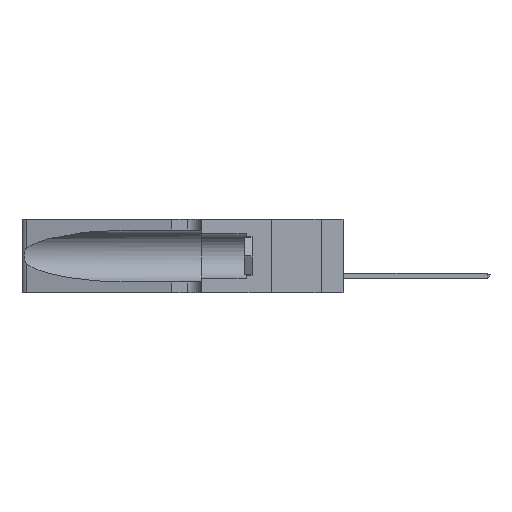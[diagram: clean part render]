
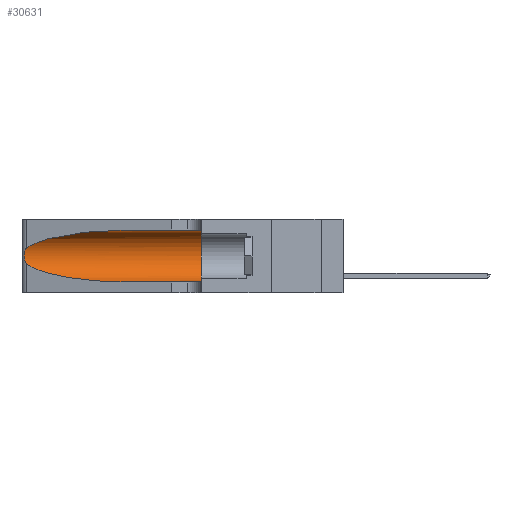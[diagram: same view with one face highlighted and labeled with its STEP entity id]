
A CAD part, left-side view. The second image highlights one B-rep face of the part: STEP entity #30631.
In plain terms, the highlighted cylindrical face has radius 3.308 mm (diameter 6.617 mm), a partial arc.
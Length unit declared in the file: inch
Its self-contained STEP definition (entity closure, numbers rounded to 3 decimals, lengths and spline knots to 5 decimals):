
#455 = ORIENTED_EDGE ( 'NONE', *, *, #36357, .T. ) ;
#565 = DIRECTION ( 'NONE',  ( 0., -1., 0. ) ) ;
#1757 = DIRECTION ( 'NONE',  ( 0., -1., 0. ) ) ;
#2036 = ORIENTED_EDGE ( 'NONE', *, *, #29687, .T. ) ;
#2436 = CARTESIAN_POINT ( 'NONE',  ( 0.26075, 1.23896, 0.178 ) ) ;
#4170 = CARTESIAN_POINT ( 'NONE',  ( 0.1305, 0.72297, 0.05475 ) ) ;
#4677 = CARTESIAN_POINT ( 'NONE',  ( 0.25555, 1.22993, 0.14849 ) ) ;
#5980 = CARTESIAN_POINT ( 'NONE',  ( 0.25789, 1.23486, 0.15765 ) ) ;
#6117 =( BOUNDED_CURVE ( )  B_SPLINE_CURVE ( 3, ( #19592, #31781, #31929, #4170 ),
 .UNSPECIFIED., .F., .T. ) 
 B_SPLINE_CURVE_WITH_KNOTS ( ( 4, 4 ),
 ( 3.44316, 4.71239 ),
 .UNSPECIFIED. ) 
 CURVE ( )  GEOMETRIC_REPRESENTATION_ITEM ( )  RATIONAL_B_SPLINE_CURVE ( ( 1., 0.87, 0.87, 1. ) ) 
 REPRESENTATION_ITEM ( '' )  );
#6506 = ORIENTED_EDGE ( 'NONE', *, *, #39464, .T. ) ;
#6916 = CARTESIAN_POINT ( 'NONE',  ( 0.25487, 1.22718, 0.22369 ) ) ;
#8922 = VERTEX_POINT ( 'NONE', #11744 ) ;
#9580 = CARTESIAN_POINT ( 'NONE',  ( 0.25639, 1.23184, 0.21858 ) ) ;
#11037 = CARTESIAN_POINT ( 'NONE',  ( 0.25856, 1.23593, 0.16098 ) ) ;
#11744 = CARTESIAN_POINT ( 'NONE',  ( 0.1305, 0.72297, 0.31525 ) ) ;
#13966 = CARTESIAN_POINT ( 'NONE',  ( 0.25487, 1.22718, 0.22369 ) ) ;
#14517 = CARTESIAN_POINT ( 'NONE',  ( 0.25854, 1.2359, 0.20912 ) ) ;
#14740 = VERTEX_POINT ( 'NONE', #47399 ) ;
#14896 = CARTESIAN_POINT ( 'NONE',  ( 0.26075, 1.23896, 0.19203 ) ) ;
#14962 = CARTESIAN_POINT ( 'NONE',  ( 0.2373, 1.15595, 0.28018 ) ) ;
#15559 = LINE ( 'NONE', #47718, #44718 ) ;
#15776 = VERTEX_POINT ( 'NONE', #25778 ) ;
#17312 = CARTESIAN_POINT ( 'NONE',  ( 0.1305, 0.72297, 0.05475 ) ) ;
#17535 = DIRECTION ( 'NONE',  ( 0., 0., 1. ) ) ;
#18070 = DIRECTION ( 'NONE',  ( 0., 0., -1. ) ) ;
#18720 = CARTESIAN_POINT ( 'NONE',  ( 0.26018, 1.23835, 0.19895 ) ) ;
#19592 = CARTESIAN_POINT ( 'NONE',  ( 0.25487, 1.22718, 0.14631 ) ) ;
#19971 = VERTEX_POINT ( 'NONE', #48031 ) ;
#20561 = CYLINDRICAL_SURFACE ( 'NONE', #24637, 0.13025 ) ;
#23439 = VECTOR ( 'NONE', #28861, 39.37008 ) ;
#24637 = AXIS2_PLACEMENT_3D ( 'NONE', #29691, #1757, #18070 ) ;
#24846 = FACE_OUTER_BOUND ( 'NONE', #45641, .T. ) ;
#25117 = CARTESIAN_POINT ( 'NONE',  ( 0.25487, 1.22718, 0.14631 ) ) ;
#25778 = CARTESIAN_POINT ( 'NONE',  ( 0.1305, 0.35, 0.31525 ) ) ;
#25941 = CIRCLE ( 'NONE', #40850, 0.13025 ) ;
#26321 = VERTEX_POINT ( 'NONE', #17312 ) ;
#26498 = CARTESIAN_POINT ( 'NONE',  ( 0.26017, 1.23833, 0.17102 ) ) ;
#27643 = ORIENTED_EDGE ( 'NONE', *, *, #34213, .F. ) ;
#28861 = DIRECTION ( 'NONE',  ( 0., -1., 0. ) ) ;
#29687 = EDGE_CURVE ( 'NONE', #8922, #14740, #35567, .T. ) ;
#29691 = CARTESIAN_POINT ( 'NONE',  ( 0.1305, 1.61858, 0.185 ) ) ;
#30631 = ADVANCED_FACE ( 'NONE', ( #24846 ), #20561, .F. ) ;
#30791 = CARTESIAN_POINT ( 'NONE',  ( 0.1305, 0.72297, 0.31525 ) ) ;
#31781 = CARTESIAN_POINT ( 'NONE',  ( 0.2373, 1.15595, 0.08982 ) ) ;
#31929 = CARTESIAN_POINT ( 'NONE',  ( 0.18966, 0.96281, 0.05475 ) ) ;
#34213 = EDGE_CURVE ( 'NONE', #8922, #15776, #15559, .T. ) ;
#34558 = ORIENTED_EDGE ( 'NONE', *, *, #35360, .F. ) ;
#35152 = CARTESIAN_POINT ( 'NONE',  ( 0.18966, 0.96281, 0.31525 ) ) ;
#35360 = EDGE_CURVE ( 'NONE', #15776, #44649, #25941, .T. ) ;
#35567 =( BOUNDED_CURVE ( )  B_SPLINE_CURVE ( 3, ( #30791, #35152, #14962, #6916 ),
 .UNSPECIFIED., .F., .T. ) 
 B_SPLINE_CURVE_WITH_KNOTS ( ( 4, 4 ),
 ( 1.5708, 2.84003 ),
 .UNSPECIFIED. ) 
 CURVE ( )  GEOMETRIC_REPRESENTATION_ITEM ( )  RATIONAL_B_SPLINE_CURVE ( ( 1., 0.87, 0.87, 1. ) ) 
 REPRESENTATION_ITEM ( '' )  );
#36357 = EDGE_CURVE ( 'NONE', #14740, #19971, #39429, .T. ) ;
#36807 = EDGE_CURVE ( 'NONE', #19971, #26321, #6117, .T. ) ;
#37091 = LINE ( 'NONE', #44902, #23439 ) ;
#39429 = B_SPLINE_CURVE_WITH_KNOTS ( 'NONE', 3,
 ( #13966, #49241, #9580, #49772, #14517, #18720, #14896, #2436, #26498, #11037, #5980, #47628, #4677, #25117 ),
 .UNSPECIFIED., .F., .F.,
 ( 4, 2, 2, 2, 2, 2, 4 ),
 ( 0., 0.00027, 0.00053, 0.00107, 0.0016, 0.00187, 0.00214 ),
 .UNSPECIFIED. ) ;
#39464 = EDGE_CURVE ( 'NONE', #26321, #44649, #37091, .T. ) ;
#39571 = CARTESIAN_POINT ( 'NONE',  ( 0.1305, 0.35, 0.05475 ) ) ;
#40850 = AXIS2_PLACEMENT_3D ( 'NONE', #49678, #41711, #17535 ) ;
#41711 = DIRECTION ( 'NONE',  ( 0., 1., 0. ) ) ;
#43765 = ORIENTED_EDGE ( 'NONE', *, *, #36807, .T. ) ;
#44649 = VERTEX_POINT ( 'NONE', #39571 ) ;
#44718 = VECTOR ( 'NONE', #565, 39.37008 ) ;
#44902 = CARTESIAN_POINT ( 'NONE',  ( 0.1305, 1.61858, 0.05475 ) ) ;
#45641 = EDGE_LOOP ( 'NONE', ( #2036, #455, #43765, #6506, #34558, #27643 ) ) ;
#47399 = CARTESIAN_POINT ( 'NONE',  ( 0.25487, 1.22718, 0.22369 ) ) ;
#47628 = CARTESIAN_POINT ( 'NONE',  ( 0.25639, 1.23186, 0.15144 ) ) ;
#47718 = CARTESIAN_POINT ( 'NONE',  ( 0.1305, 1.61858, 0.31525 ) ) ;
#48031 = CARTESIAN_POINT ( 'NONE',  ( 0.25487, 1.22718, 0.14631 ) ) ;
#49241 = CARTESIAN_POINT ( 'NONE',  ( 0.25555, 1.22994, 0.2215 ) ) ;
#49678 = CARTESIAN_POINT ( 'NONE',  ( 0.1305, 0.35, 0.185 ) ) ;
#49772 = CARTESIAN_POINT ( 'NONE',  ( 0.25787, 1.23484, 0.2124 ) ) ;
